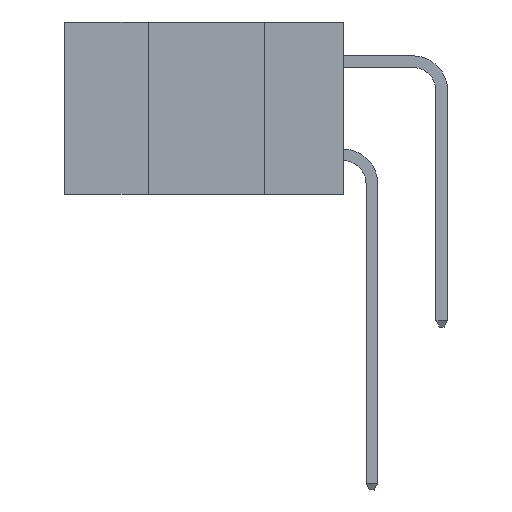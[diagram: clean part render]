
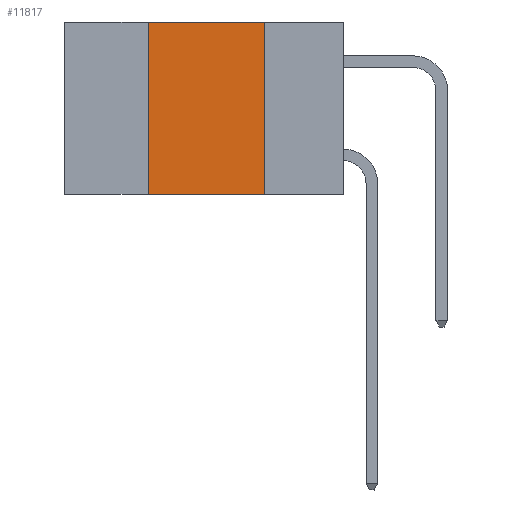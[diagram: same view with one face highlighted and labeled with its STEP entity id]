
A CAD part, left-side view. The second image highlights one B-rep face of the part: STEP entity #11817.
In plain terms, the highlighted planar face has unit normal (-1, 0, 0).
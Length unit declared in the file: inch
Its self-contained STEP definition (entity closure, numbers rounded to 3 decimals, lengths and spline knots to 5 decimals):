
#426 = CARTESIAN_POINT ( 'NONE',  ( 0., 0.17, 0. ) ) ;
#955 = DIRECTION ( 'NONE',  ( 0., -1., 0. ) ) ;
#1166 = LINE ( 'NONE', #17550, #19328 ) ;
#1236 = DIRECTION ( 'NONE',  ( 0., -1., 0. ) ) ;
#1798 = AXIS2_PLACEMENT_3D ( 'NONE', #9176, #25735, #11531 ) ;
#2988 = CARTESIAN_POINT ( 'NONE',  ( 0., 0.42, 0. ) ) ;
#5159 = VERTEX_POINT ( 'NONE', #426 ) ;
#6367 = LINE ( 'NONE', #21934, #29265 ) ;
#6692 = EDGE_CURVE ( 'NONE', #19868, #5159, #1166, .T. ) ;
#7476 = CARTESIAN_POINT ( 'NONE',  ( 0., 0.17, -0.37 ) ) ;
#7774 = DIRECTION ( 'NONE',  ( 0., 0., -1. ) ) ;
#8029 = LINE ( 'NONE', #13020, #14263 ) ;
#8736 = VERTEX_POINT ( 'NONE', #12951 ) ;
#9176 = CARTESIAN_POINT ( 'NONE',  ( 0., 0.6, 0. ) ) ;
#10089 = ORIENTED_EDGE ( 'NONE', *, *, #26970, .F. ) ;
#11531 = DIRECTION ( 'NONE',  ( 0., 0., -1. ) ) ;
#11817 = ADVANCED_FACE ( 'NONE', ( #28100 ), #20987, .F. ) ;
#12951 = CARTESIAN_POINT ( 'NONE',  ( 0., 0.42, -0.37 ) ) ;
#13020 = CARTESIAN_POINT ( 'NONE',  ( 0., 0.6, -0.37 ) ) ;
#14263 = VECTOR ( 'NONE', #1236, 39.37008 ) ;
#15630 = ORIENTED_EDGE ( 'NONE', *, *, #6692, .F. ) ;
#16370 = ORIENTED_EDGE ( 'NONE', *, *, #23628, .T. ) ;
#17175 = DIRECTION ( 'NONE',  ( 0., 0., 1. ) ) ;
#17550 = CARTESIAN_POINT ( 'NONE',  ( 0., 0.6, 0. ) ) ;
#18135 = VERTEX_POINT ( 'NONE', #7476 ) ;
#19328 = VECTOR ( 'NONE', #955, 39.37008 ) ;
#19868 = VERTEX_POINT ( 'NONE', #21651 ) ;
#20987 = PLANE ( 'NONE',  #1798 ) ;
#21651 = CARTESIAN_POINT ( 'NONE',  ( 0., 0.42, 0. ) ) ;
#21934 = CARTESIAN_POINT ( 'NONE',  ( 0., 0.17, 0. ) ) ;
#23628 = EDGE_CURVE ( 'NONE', #8736, #18135, #8029, .T. ) ;
#24009 = EDGE_LOOP ( 'NONE', ( #27518, #15630, #10089, #16370 ) ) ;
#24714 = LINE ( 'NONE', #2988, #25453 ) ;
#25453 = VECTOR ( 'NONE', #17175, 39.37008 ) ;
#25735 = DIRECTION ( 'NONE',  ( 1., 0., 0. ) ) ;
#26970 = EDGE_CURVE ( 'NONE', #8736, #19868, #24714, .T. ) ;
#27518 = ORIENTED_EDGE ( 'NONE', *, *, #30503, .F. ) ;
#28100 = FACE_OUTER_BOUND ( 'NONE', #24009, .T. ) ;
#29265 = VECTOR ( 'NONE', #7774, 39.37008 ) ;
#30503 = EDGE_CURVE ( 'NONE', #5159, #18135, #6367, .T. ) ;
